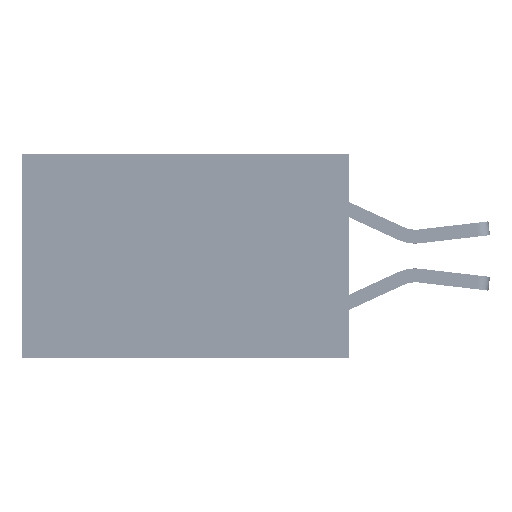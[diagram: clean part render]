
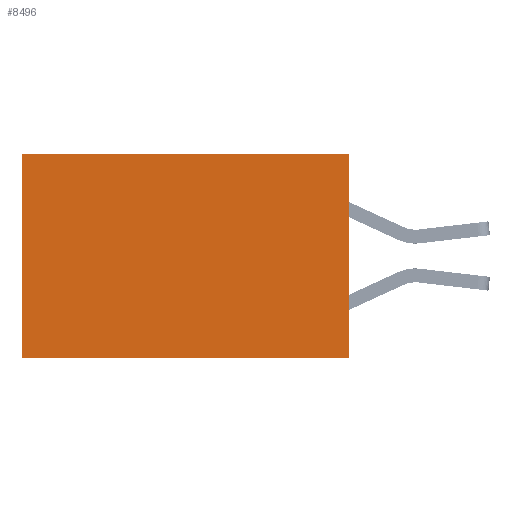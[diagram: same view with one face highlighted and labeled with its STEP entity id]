
A CAD part, left-side view. The second image highlights one B-rep face of the part: STEP entity #8496.
In plain terms, the highlighted planar face has unit normal (-1, 0, 0).
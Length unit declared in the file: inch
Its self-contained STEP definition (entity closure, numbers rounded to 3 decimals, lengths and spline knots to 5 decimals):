
#357 = DIRECTION ( 'NONE',  ( 0., 1., 0. ) ) ;
#577 = VERTEX_POINT ( 'NONE', #10184 ) ;
#2701 = CARTESIAN_POINT ( 'NONE',  ( 0.277, 0.59, -0.37 ) ) ;
#2833 = CARTESIAN_POINT ( 'NONE',  ( 0.277, 0., -0.37 ) ) ;
#3264 = EDGE_CURVE ( 'NONE', #32385, #11168, #14201, .T. ) ;
#4031 = EDGE_CURVE ( 'NONE', #5215, #577, #18992, .T. ) ;
#4246 = VECTOR ( 'NONE', #22571, 39.37008 ) ;
#5215 = VERTEX_POINT ( 'NONE', #26616 ) ;
#5465 = EDGE_CURVE ( 'NONE', #5215, #32385, #11225, .T. ) ;
#7858 = CARTESIAN_POINT ( 'NONE',  ( 0.277, 0.59, 0. ) ) ;
#8496 = ADVANCED_FACE ( 'NONE', ( #20781 ), #28856, .F. ) ;
#10184 = CARTESIAN_POINT ( 'NONE',  ( 0.277, 0., -0.37 ) ) ;
#10842 = CARTESIAN_POINT ( 'NONE',  ( 0.277, 0., -0.37 ) ) ;
#11168 = VERTEX_POINT ( 'NONE', #2701 ) ;
#11225 = LINE ( 'NONE', #22544, #4246 ) ;
#11279 = VECTOR ( 'NONE', #26399, 39.37008 ) ;
#13367 = DIRECTION ( 'NONE',  ( 1., 0., 0. ) ) ;
#14201 = LINE ( 'NONE', #29729, #21082 ) ;
#14262 = LINE ( 'NONE', #10842, #26371 ) ;
#14280 = ORIENTED_EDGE ( 'NONE', *, *, #14409, .F. ) ;
#14409 = EDGE_CURVE ( 'NONE', #577, #11168, #14262, .T. ) ;
#16761 = AXIS2_PLACEMENT_3D ( 'NONE', #2833, #13367, #31446 ) ;
#18992 = LINE ( 'NONE', #27062, #11279 ) ;
#20111 = ORIENTED_EDGE ( 'NONE', *, *, #4031, .F. ) ;
#20781 = FACE_OUTER_BOUND ( 'NONE', #22662, .T. ) ;
#21082 = VECTOR ( 'NONE', #29662, 39.37008 ) ;
#22544 = CARTESIAN_POINT ( 'NONE',  ( 0.277, 0., 0. ) ) ;
#22571 = DIRECTION ( 'NONE',  ( 0., 1., 0. ) ) ;
#22662 = EDGE_LOOP ( 'NONE', ( #30995, #14280, #20111, #29436 ) ) ;
#26371 = VECTOR ( 'NONE', #357, 39.37008 ) ;
#26399 = DIRECTION ( 'NONE',  ( 0., 0., -1. ) ) ;
#26616 = CARTESIAN_POINT ( 'NONE',  ( 0.277, 0., 0. ) ) ;
#27062 = CARTESIAN_POINT ( 'NONE',  ( 0.277, 0., -0.37 ) ) ;
#28856 = PLANE ( 'NONE',  #16761 ) ;
#29436 = ORIENTED_EDGE ( 'NONE', *, *, #5465, .T. ) ;
#29662 = DIRECTION ( 'NONE',  ( 0., 0., -1. ) ) ;
#29729 = CARTESIAN_POINT ( 'NONE',  ( 0.277, 0.59, -0.37 ) ) ;
#30995 = ORIENTED_EDGE ( 'NONE', *, *, #3264, .T. ) ;
#31446 = DIRECTION ( 'NONE',  ( 0., 0., -1. ) ) ;
#32385 = VERTEX_POINT ( 'NONE', #7858 ) ;
